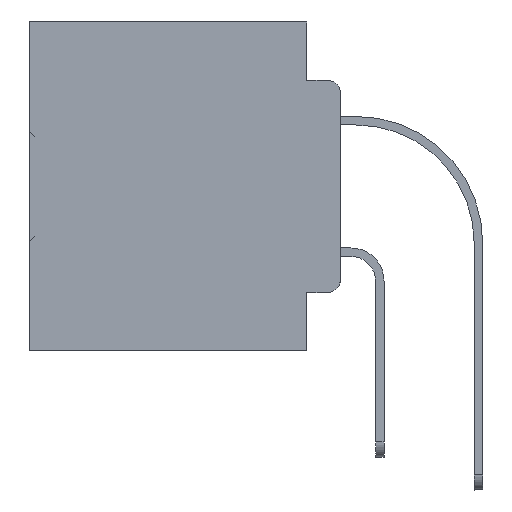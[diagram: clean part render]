
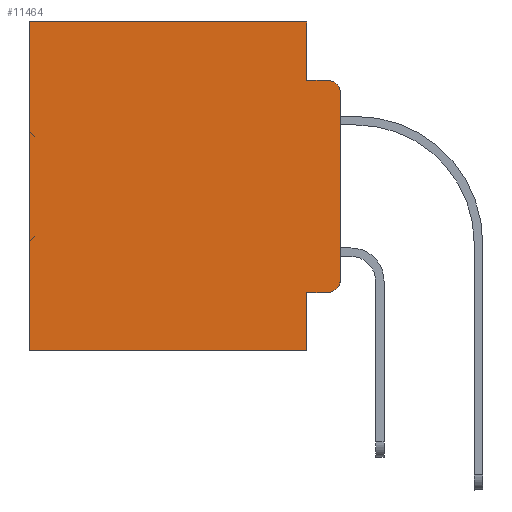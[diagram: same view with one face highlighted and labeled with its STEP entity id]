
A CAD part, left-side view. The second image highlights one B-rep face of the part: STEP entity #11464.
In plain terms, the highlighted planar face has unit normal (-1, 0, 0).
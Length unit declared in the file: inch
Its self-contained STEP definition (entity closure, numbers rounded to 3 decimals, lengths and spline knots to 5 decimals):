
#784 = ORIENTED_EDGE ( 'NONE', *, *, #27907, .F. ) ;
#1191 = EDGE_CURVE ( 'NONE', #31869, #33035, #36895, .T. ) ;
#1424 = EDGE_CURVE ( 'NONE', #33035, #22241, #20443, .T. ) ;
#1533 = LINE ( 'NONE', #20744, #16982 ) ;
#1823 = VERTEX_POINT ( 'NONE', #10644 ) ;
#2697 = CARTESIAN_POINT ( 'NONE',  ( 0.298, 0.473, -0.5 ) ) ;
#2992 = DIRECTION ( 'NONE',  ( -1., 0., 0. ) ) ;
#3797 = AXIS2_PLACEMENT_3D ( 'NONE', #30351, #2992, #5824 ) ;
#4369 = ORIENTED_EDGE ( 'NONE', *, *, #1191, .F. ) ;
#4727 = ORIENTED_EDGE ( 'NONE', *, *, #21635, .F. ) ;
#5209 = LINE ( 'NONE', #8648, #12408 ) ;
#5824 = DIRECTION ( 'NONE',  ( 0., 0., -1. ) ) ;
#6198 = VERTEX_POINT ( 'NONE', #15802 ) ;
#6540 = CARTESIAN_POINT ( 'NONE',  ( 0.298, 0.02, -0.0885 ) ) ;
#7587 = VERTEX_POINT ( 'NONE', #2697 ) ;
#8221 = VECTOR ( 'NONE', #30807, 39.37008 ) ;
#8648 = CARTESIAN_POINT ( 'NONE',  ( 0.298, 0., -0.5 ) ) ;
#8674 = DIRECTION ( 'NONE',  ( 0., 0., -1. ) ) ;
#8813 = ORIENTED_EDGE ( 'NONE', *, *, #25331, .T. ) ;
#8880 = DIRECTION ( 'NONE',  ( 1., 0., 0. ) ) ;
#9292 = CARTESIAN_POINT ( 'NONE',  ( 0.298, 0.051, -0.4115 ) ) ;
#9595 = AXIS2_PLACEMENT_3D ( 'NONE', #31235, #22489, #37524 ) ;
#9955 = CARTESIAN_POINT ( 'NONE',  ( 0.298, 0., 0. ) ) ;
#10644 = CARTESIAN_POINT ( 'NONE',  ( 0.298, 0.02, -0.4115 ) ) ;
#11108 = DIRECTION ( 'NONE',  ( 0., 1., 0. ) ) ;
#11464 = ADVANCED_FACE ( 'NONE', ( #29769 ), #26748, .F. ) ;
#11600 = VERTEX_POINT ( 'NONE', #9292 ) ;
#11630 = VERTEX_POINT ( 'NONE', #21832 ) ;
#11720 = LINE ( 'NONE', #36462, #25138 ) ;
#11769 = CARTESIAN_POINT ( 'NONE',  ( 0.298, 0.051, 0. ) ) ;
#12174 = EDGE_CURVE ( 'NONE', #16658, #7587, #34968, .T. ) ;
#12408 = VECTOR ( 'NONE', #11108, 39.37008 ) ;
#13678 = VECTOR ( 'NONE', #32135, 39.37008 ) ;
#14586 = CARTESIAN_POINT ( 'NONE',  ( 0.298, 0., 0. ) ) ;
#14963 = LINE ( 'NONE', #26533, #20153 ) ;
#15802 = CARTESIAN_POINT ( 'NONE',  ( 0.298, 0., -0.3915 ) ) ;
#16658 = VERTEX_POINT ( 'NONE', #25576 ) ;
#16982 = VECTOR ( 'NONE', #33135, 39.37008 ) ;
#17933 = VECTOR ( 'NONE', #27310, 39.37008 ) ;
#18542 = EDGE_CURVE ( 'NONE', #1823, #6198, #25117, .T. ) ;
#18761 = AXIS2_PLACEMENT_3D ( 'NONE', #14586, #8880, #33245 ) ;
#19136 = ORIENTED_EDGE ( 'NONE', *, *, #18542, .T. ) ;
#19750 = CARTESIAN_POINT ( 'NONE',  ( 0.298, 0.473, 0. ) ) ;
#20153 = VECTOR ( 'NONE', #32642, 39.37008 ) ;
#20443 = LINE ( 'NONE', #39497, #17933 ) ;
#20717 = CARTESIAN_POINT ( 'NONE',  ( 0.298, 0.051, -0.5 ) ) ;
#20744 = CARTESIAN_POINT ( 'NONE',  ( 0.298, 0.051, -0.4115 ) ) ;
#21467 = CARTESIAN_POINT ( 'NONE',  ( 0.298, 0.051, 0. ) ) ;
#21635 = EDGE_CURVE ( 'NONE', #31311, #7587, #5209, .T. ) ;
#21832 = CARTESIAN_POINT ( 'NONE',  ( 0.298, 0., -0.1085 ) ) ;
#22241 = VERTEX_POINT ( 'NONE', #6540 ) ;
#22489 = DIRECTION ( 'NONE',  ( -1., 0., 0. ) ) ;
#23325 = CARTESIAN_POINT ( 'NONE',  ( 0.298, 0.051, -0.0885 ) ) ;
#24173 = EDGE_CURVE ( 'NONE', #31869, #16658, #34878, .T. ) ;
#25117 = CIRCLE ( 'NONE', #9595, 0.02 ) ;
#25138 = VECTOR ( 'NONE', #8674, 39.37008 ) ;
#25331 = EDGE_CURVE ( 'NONE', #11630, #22241, #32957, .T. ) ;
#25576 = CARTESIAN_POINT ( 'NONE',  ( 0.298, 0.473, 0. ) ) ;
#26533 = CARTESIAN_POINT ( 'NONE',  ( 0.298, 0., 0. ) ) ;
#26748 = PLANE ( 'NONE',  #18761 ) ;
#27310 = DIRECTION ( 'NONE',  ( 0., -1., 0. ) ) ;
#27907 = EDGE_CURVE ( 'NONE', #11630, #6198, #14963, .T. ) ;
#28374 = DIRECTION ( 'NONE',  ( 0., 1., 0. ) ) ;
#28732 = EDGE_CURVE ( 'NONE', #11600, #1823, #1533, .T. ) ;
#28782 = EDGE_LOOP ( 'NONE', ( #784, #8813, #32590, #4369, #32132, #37191, #4727, #37421, #32232, #19136 ) ) ;
#29620 = VECTOR ( 'NONE', #28374, 39.37008 ) ;
#29769 = FACE_OUTER_BOUND ( 'NONE', #28782, .T. ) ;
#30351 = CARTESIAN_POINT ( 'NONE',  ( 0.298, 0.02, -0.1085 ) ) ;
#30807 = DIRECTION ( 'NONE',  ( 0., 0., -1. ) ) ;
#31235 = CARTESIAN_POINT ( 'NONE',  ( 0.298, 0.02, -0.3915 ) ) ;
#31311 = VERTEX_POINT ( 'NONE', #20717 ) ;
#31869 = VERTEX_POINT ( 'NONE', #11769 ) ;
#32132 = ORIENTED_EDGE ( 'NONE', *, *, #24173, .T. ) ;
#32135 = DIRECTION ( 'NONE',  ( 0., 0., -1. ) ) ;
#32232 = ORIENTED_EDGE ( 'NONE', *, *, #28732, .T. ) ;
#32590 = ORIENTED_EDGE ( 'NONE', *, *, #1424, .F. ) ;
#32642 = DIRECTION ( 'NONE',  ( 0., 0., -1. ) ) ;
#32957 = CIRCLE ( 'NONE', #3797, 0.02 ) ;
#33035 = VERTEX_POINT ( 'NONE', #23325 ) ;
#33135 = DIRECTION ( 'NONE',  ( 0., -1., 0. ) ) ;
#33245 = DIRECTION ( 'NONE',  ( 0., 0., -1. ) ) ;
#34878 = LINE ( 'NONE', #9955, #29620 ) ;
#34968 = LINE ( 'NONE', #19750, #13678 ) ;
#35979 = EDGE_CURVE ( 'NONE', #11600, #31311, #11720, .T. ) ;
#36462 = CARTESIAN_POINT ( 'NONE',  ( 0.298, 0.051, 0. ) ) ;
#36895 = LINE ( 'NONE', #21467, #8221 ) ;
#37191 = ORIENTED_EDGE ( 'NONE', *, *, #12174, .T. ) ;
#37421 = ORIENTED_EDGE ( 'NONE', *, *, #35979, .F. ) ;
#37524 = DIRECTION ( 'NONE',  ( 0., 0., -1. ) ) ;
#39497 = CARTESIAN_POINT ( 'NONE',  ( 0.298, 0.051, -0.0885 ) ) ;
